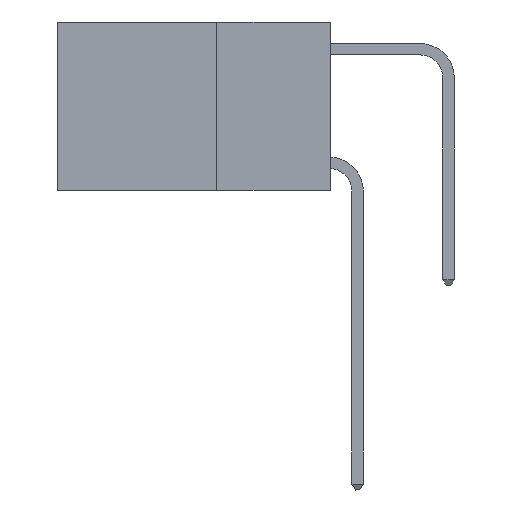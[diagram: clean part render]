
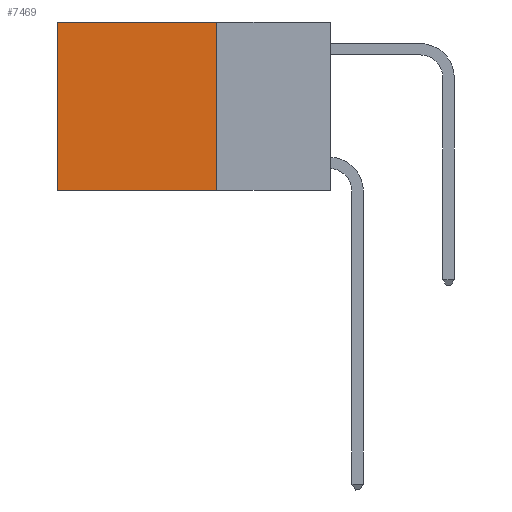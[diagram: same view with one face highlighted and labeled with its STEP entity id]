
A CAD part, left-side view. The second image highlights one B-rep face of the part: STEP entity #7469.
In plain terms, the highlighted planar face has unit normal (-1, 0, 0).
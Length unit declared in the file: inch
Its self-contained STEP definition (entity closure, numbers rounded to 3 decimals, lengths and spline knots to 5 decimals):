
#1064 = VERTEX_POINT ( 'NONE', #6866 ) ;
#2075 = VECTOR ( 'NONE', #8849, 39.37008 ) ;
#2570 = EDGE_LOOP ( 'NONE', ( #2735, #14078, #10011, #13151 ) ) ;
#2735 = ORIENTED_EDGE ( 'NONE', *, *, #13626, .T. ) ;
#3067 = VERTEX_POINT ( 'NONE', #9184 ) ;
#3261 = FACE_OUTER_BOUND ( 'NONE', #2570, .T. ) ;
#4231 = VERTEX_POINT ( 'NONE', #10858 ) ;
#4582 = DIRECTION ( 'NONE',  ( 1., 0., 0. ) ) ;
#6866 = CARTESIAN_POINT ( 'NONE',  ( 0.2625, 0.6, 0. ) ) ;
#7469 = ADVANCED_FACE ( 'NONE', ( #3261 ), #11187, .F. ) ;
#7601 = CARTESIAN_POINT ( 'NONE',  ( 0.2625, 0.25, 0. ) ) ;
#7628 = CARTESIAN_POINT ( 'NONE',  ( 0.2625, 0.25, -0.37 ) ) ;
#7953 = DIRECTION ( 'NONE',  ( 0., 0., -1. ) ) ;
#8541 = VERTEX_POINT ( 'NONE', #7628 ) ;
#8849 = DIRECTION ( 'NONE',  ( 0., 0., -1. ) ) ;
#8935 = LINE ( 'NONE', #10287, #16449 ) ;
#9181 = LINE ( 'NONE', #9326, #15059 ) ;
#9184 = CARTESIAN_POINT ( 'NONE',  ( 0.2625, 0.6, -0.37 ) ) ;
#9326 = CARTESIAN_POINT ( 'NONE',  ( 0.2625, 0.25, -0.37 ) ) ;
#9568 = VECTOR ( 'NONE', #7953, 39.37008 ) ;
#9942 = LINE ( 'NONE', #7601, #2075 ) ;
#10011 = ORIENTED_EDGE ( 'NONE', *, *, #13101, .F. ) ;
#10287 = CARTESIAN_POINT ( 'NONE',  ( 0.2625, 0.25, 0. ) ) ;
#10516 = CARTESIAN_POINT ( 'NONE',  ( 0.2625, 0.6, 0. ) ) ;
#10858 = CARTESIAN_POINT ( 'NONE',  ( 0.2625, 0.25, 0. ) ) ;
#11109 = DIRECTION ( 'NONE',  ( 0., 0., -1. ) ) ;
#11187 = PLANE ( 'NONE',  #12952 ) ;
#12779 = LINE ( 'NONE', #10516, #9568 ) ;
#12952 = AXIS2_PLACEMENT_3D ( 'NONE', #16255, #4582, #11109 ) ;
#13061 = EDGE_CURVE ( 'NONE', #4231, #1064, #8935, .T. ) ;
#13101 = EDGE_CURVE ( 'NONE', #4231, #8541, #9942, .T. ) ;
#13151 = ORIENTED_EDGE ( 'NONE', *, *, #13061, .T. ) ;
#13626 = EDGE_CURVE ( 'NONE', #1064, #3067, #12779, .T. ) ;
#14078 = ORIENTED_EDGE ( 'NONE', *, *, #14326, .F. ) ;
#14326 = EDGE_CURVE ( 'NONE', #8541, #3067, #9181, .T. ) ;
#14561 = DIRECTION ( 'NONE',  ( 0., 1., 0. ) ) ;
#15059 = VECTOR ( 'NONE', #14561, 39.37008 ) ;
#16255 = CARTESIAN_POINT ( 'NONE',  ( 0.2625, 0.25, 0. ) ) ;
#16449 = VECTOR ( 'NONE', #16710, 39.37008 ) ;
#16710 = DIRECTION ( 'NONE',  ( 0., 1., 0. ) ) ;
